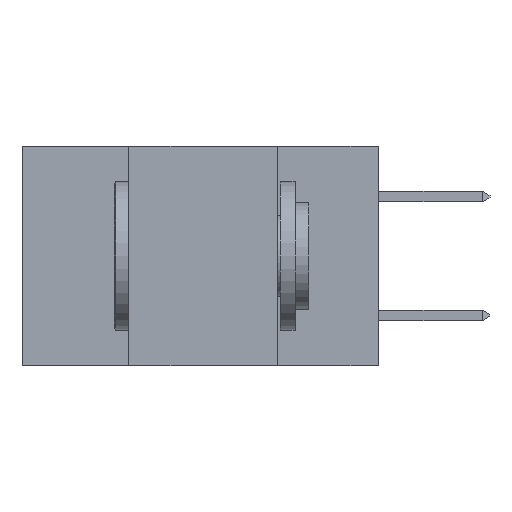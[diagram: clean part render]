
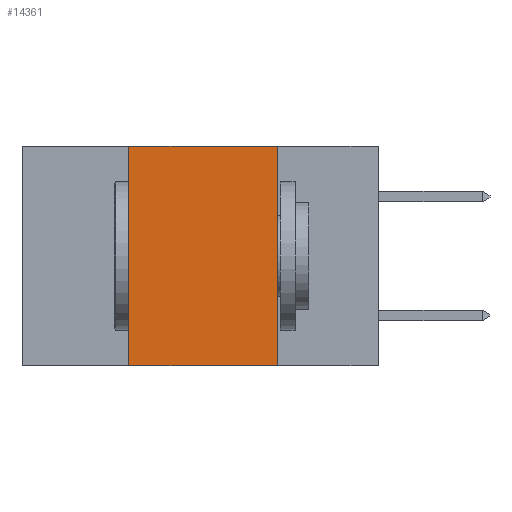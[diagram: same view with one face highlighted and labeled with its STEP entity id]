
A CAD part, left-side view. The second image highlights one B-rep face of the part: STEP entity #14361.
In plain terms, the highlighted planar face has unit normal (-1, 0, 0).
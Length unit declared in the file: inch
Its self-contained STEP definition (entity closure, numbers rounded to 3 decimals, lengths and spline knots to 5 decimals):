
#179 = EDGE_CURVE ( 'NONE', #4823, #13455, #12980, .T. ) ;
#914 = CARTESIAN_POINT ( 'NONE',  ( 0., 0.42, 0. ) ) ;
#1260 = CARTESIAN_POINT ( 'NONE',  ( 0., 0.17, 0. ) ) ;
#1428 = VECTOR ( 'NONE', #13414, 39.37008 ) ;
#1763 = ORIENTED_EDGE ( 'NONE', *, *, #12347, .T. ) ;
#2567 = CARTESIAN_POINT ( 'NONE',  ( 0., 0.42, -0.37 ) ) ;
#2789 = CARTESIAN_POINT ( 'NONE',  ( 0., 0.6, 0. ) ) ;
#2870 = VECTOR ( 'NONE', #12393, 39.37008 ) ;
#3259 = LINE ( 'NONE', #11347, #2870 ) ;
#4029 = DIRECTION ( 'NONE',  ( 1., 0., 0. ) ) ;
#4823 = VERTEX_POINT ( 'NONE', #914 ) ;
#5200 = ORIENTED_EDGE ( 'NONE', *, *, #179, .F. ) ;
#5766 = CARTESIAN_POINT ( 'NONE',  ( 0., 0.17, -0.37 ) ) ;
#6818 = FACE_OUTER_BOUND ( 'NONE', #8600, .T. ) ;
#7542 = DIRECTION ( 'NONE',  ( 0., -1., 0. ) ) ;
#7781 = EDGE_CURVE ( 'NONE', #13455, #11774, #10791, .T. ) ;
#8083 = CARTESIAN_POINT ( 'NONE',  ( 0., 0.42, 0. ) ) ;
#8307 = ORIENTED_EDGE ( 'NONE', *, *, #11132, .F. ) ;
#8600 = EDGE_LOOP ( 'NONE', ( #10946, #5200, #8307, #1763 ) ) ;
#8643 = VERTEX_POINT ( 'NONE', #2567 ) ;
#8762 = AXIS2_PLACEMENT_3D ( 'NONE', #2789, #4029, #12038 ) ;
#9888 = PLANE ( 'NONE',  #8762 ) ;
#9909 = CARTESIAN_POINT ( 'NONE',  ( 0., 0.6, 0. ) ) ;
#10791 = LINE ( 'NONE', #1260, #1428 ) ;
#10946 = ORIENTED_EDGE ( 'NONE', *, *, #7781, .F. ) ;
#11132 = EDGE_CURVE ( 'NONE', #8643, #4823, #12443, .T. ) ;
#11347 = CARTESIAN_POINT ( 'NONE',  ( 0., 0.6, -0.37 ) ) ;
#11416 = DIRECTION ( 'NONE',  ( 0., 0., 1. ) ) ;
#11774 = VERTEX_POINT ( 'NONE', #5766 ) ;
#12038 = DIRECTION ( 'NONE',  ( 0., 0., -1. ) ) ;
#12347 = EDGE_CURVE ( 'NONE', #8643, #11774, #3259, .T. ) ;
#12393 = DIRECTION ( 'NONE',  ( 0., -1., 0. ) ) ;
#12443 = LINE ( 'NONE', #8083, #14573 ) ;
#12639 = VECTOR ( 'NONE', #7542, 39.37008 ) ;
#12980 = LINE ( 'NONE', #9909, #12639 ) ;
#13363 = CARTESIAN_POINT ( 'NONE',  ( 0., 0.17, 0. ) ) ;
#13414 = DIRECTION ( 'NONE',  ( 0., 0., -1. ) ) ;
#13455 = VERTEX_POINT ( 'NONE', #13363 ) ;
#14361 = ADVANCED_FACE ( 'NONE', ( #6818 ), #9888, .F. ) ;
#14573 = VECTOR ( 'NONE', #11416, 39.37008 ) ;
